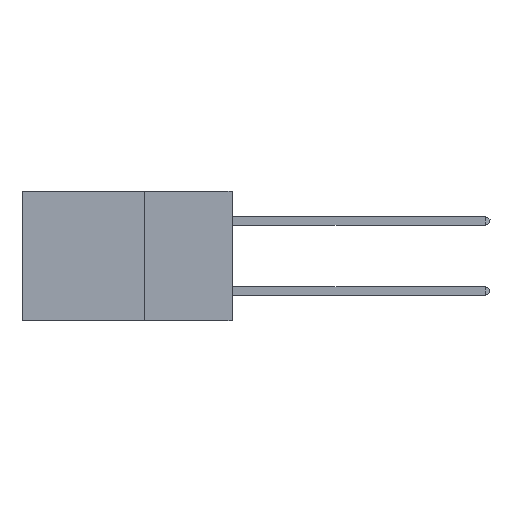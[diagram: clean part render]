
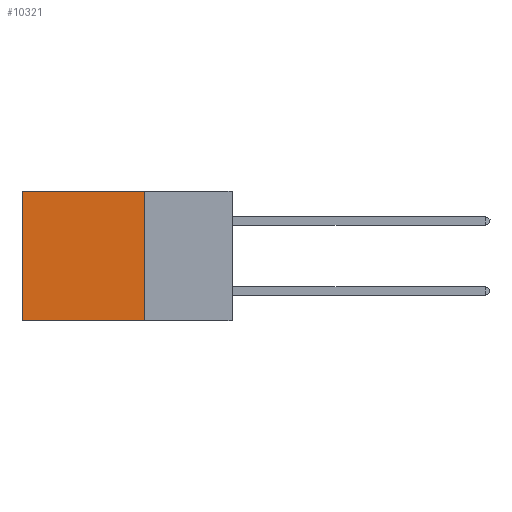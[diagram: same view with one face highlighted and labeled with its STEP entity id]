
A CAD part, left-side view. The second image highlights one B-rep face of the part: STEP entity #10321.
In plain terms, the highlighted planar face has unit normal (-1, 0, 0).
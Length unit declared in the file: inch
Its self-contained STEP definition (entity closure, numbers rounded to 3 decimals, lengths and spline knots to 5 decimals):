
#1577 = DIRECTION ( 'NONE',  ( 0., 0., -1. ) ) ;
#1738 = CARTESIAN_POINT ( 'NONE',  ( 0.2875, 0.25, 0. ) ) ;
#3665 = VERTEX_POINT ( 'NONE', #8055 ) ;
#4055 = EDGE_CURVE ( 'NONE', #38729, #13086, #16344, .T. ) ;
#5249 = LINE ( 'NONE', #19541, #39547 ) ;
#7991 = VECTOR ( 'NONE', #28665, 39.37008 ) ;
#8055 = CARTESIAN_POINT ( 'NONE',  ( 0.2875, 0.25, 0. ) ) ;
#10321 = ADVANCED_FACE ( 'NONE', ( #14452 ), #26401, .F. ) ;
#12727 = LINE ( 'NONE', #19814, #7991 ) ;
#13086 = VERTEX_POINT ( 'NONE', #17144 ) ;
#13756 = CARTESIAN_POINT ( 'NONE',  ( 0.2875, 0.25, -0.37 ) ) ;
#14452 = FACE_OUTER_BOUND ( 'NONE', #28324, .T. ) ;
#16055 = AXIS2_PLACEMENT_3D ( 'NONE', #1738, #41315, #1577 ) ;
#16344 = LINE ( 'NONE', #36676, #27763 ) ;
#16731 = VECTOR ( 'NONE', #18361, 39.37008 ) ;
#17144 = CARTESIAN_POINT ( 'NONE',  ( 0.2875, 0.6, -0.37 ) ) ;
#17204 = ORIENTED_EDGE ( 'NONE', *, *, #25545, .T. ) ;
#17288 = CARTESIAN_POINT ( 'NONE',  ( 0.2875, 0.25, 0. ) ) ;
#18361 = DIRECTION ( 'NONE',  ( 0., 1., 0. ) ) ;
#19541 = CARTESIAN_POINT ( 'NONE',  ( 0.2875, 0.6, 0. ) ) ;
#19814 = CARTESIAN_POINT ( 'NONE',  ( 0.2875, 0.25, 0. ) ) ;
#24419 = CARTESIAN_POINT ( 'NONE',  ( 0.2875, 0.6, 0. ) ) ;
#25545 = EDGE_CURVE ( 'NONE', #3665, #40538, #36487, .T. ) ;
#25929 = EDGE_CURVE ( 'NONE', #40538, #13086, #5249, .T. ) ;
#26401 = PLANE ( 'NONE',  #16055 ) ;
#27763 = VECTOR ( 'NONE', #36827, 39.37008 ) ;
#28324 = EDGE_LOOP ( 'NONE', ( #31836, #30674, #36140, #17204 ) ) ;
#28665 = DIRECTION ( 'NONE',  ( 0., 0., -1. ) ) ;
#30674 = ORIENTED_EDGE ( 'NONE', *, *, #4055, .F. ) ;
#31322 = EDGE_CURVE ( 'NONE', #3665, #38729, #12727, .T. ) ;
#31836 = ORIENTED_EDGE ( 'NONE', *, *, #25929, .T. ) ;
#36140 = ORIENTED_EDGE ( 'NONE', *, *, #31322, .F. ) ;
#36487 = LINE ( 'NONE', #17288, #16731 ) ;
#36676 = CARTESIAN_POINT ( 'NONE',  ( 0.2875, 0.25, -0.37 ) ) ;
#36827 = DIRECTION ( 'NONE',  ( 0., 1., 0. ) ) ;
#38729 = VERTEX_POINT ( 'NONE', #13756 ) ;
#39547 = VECTOR ( 'NONE', #42334, 39.37008 ) ;
#40538 = VERTEX_POINT ( 'NONE', #24419 ) ;
#41315 = DIRECTION ( 'NONE',  ( 1., 0., 0. ) ) ;
#42334 = DIRECTION ( 'NONE',  ( 0., 0., -1. ) ) ;
